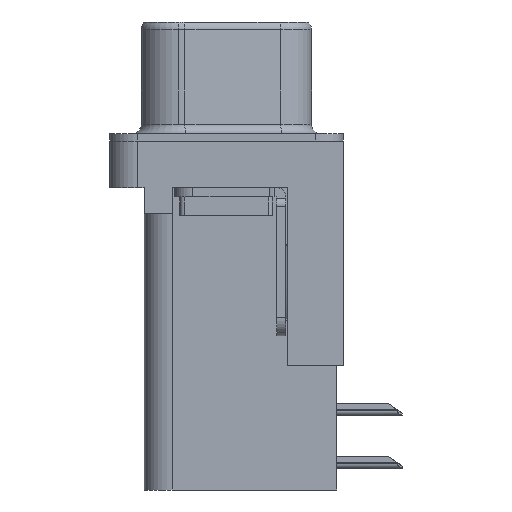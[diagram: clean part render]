
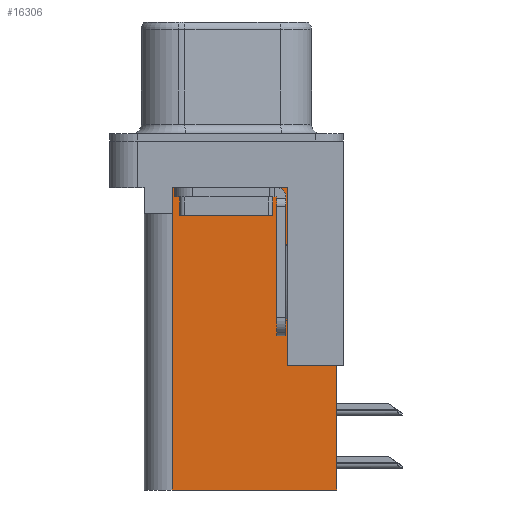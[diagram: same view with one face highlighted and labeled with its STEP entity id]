
A CAD part, left-side view. The second image highlights one B-rep face of the part: STEP entity #16306.
In plain terms, the highlighted planar face has unit normal (-1, 0, 0).
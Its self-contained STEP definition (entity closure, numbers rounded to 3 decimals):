
#5 = CARTESIAN_POINT ( 'NONE',  ( 3.7, -3.295, -18.76 ) ) ;
#32 = ORIENTED_EDGE ( 'NONE', *, *, #1229, .F. ) ;
#220 = ORIENTED_EDGE ( 'NONE', *, *, #6097, .T. ) ;
#308 = VERTEX_POINT ( 'NONE', #11061 ) ;
#889 = VERTEX_POINT ( 'NONE', #10891 ) ;
#1229 = EDGE_CURVE ( 'NONE', #1233, #20157, #14861, .T. ) ;
#1233 = VERTEX_POINT ( 'NONE', #16922 ) ;
#1778 = VERTEX_POINT ( 'NONE', #19471 ) ;
#2435 = DIRECTION ( 'NONE',  ( 0., 0., -1. ) ) ;
#2873 = DIRECTION ( 'NONE',  ( 0., 1., 0. ) ) ;
#2878 = VECTOR ( 'NONE', #2435, 1000. ) ;
#3005 = LINE ( 'NONE', #23291, #2878 ) ;
#3459 = CARTESIAN_POINT ( 'NONE',  ( 3.7, 2.925, -18.76 ) ) ;
#4246 = DIRECTION ( 'NONE',  ( 0., 1., 0. ) ) ;
#4630 = CARTESIAN_POINT ( 'NONE',  ( 3.7, -5.925, -18.76 ) ) ;
#5205 = VECTOR ( 'NONE', #12821, 1000. ) ;
#6097 = EDGE_CURVE ( 'NONE', #1233, #308, #6767, .T. ) ;
#6763 = VECTOR ( 'NONE', #7307, 1000. ) ;
#6767 = LINE ( 'NONE', #13098, #6763 ) ;
#7030 = ORIENTED_EDGE ( 'NONE', *, *, #12624, .T. ) ;
#7238 = DIRECTION ( 'NONE',  ( 0., 1., 0. ) ) ;
#7307 = DIRECTION ( 'NONE',  ( 0., 1., 0. ) ) ;
#7654 = CARTESIAN_POINT ( 'NONE',  ( 3.7, 2.925, -18.76 ) ) ;
#9260 = CARTESIAN_POINT ( 'NONE',  ( 3.7, 2.925, -3.9 ) ) ;
#9884 = ORIENTED_EDGE ( 'NONE', *, *, #19388, .T. ) ;
#10268 = VERTEX_POINT ( 'NONE', #9260 ) ;
#10859 = ORIENTED_EDGE ( 'NONE', *, *, #14201, .T. ) ;
#10891 = CARTESIAN_POINT ( 'NONE',  ( 3.7, 2.895, -2.5 ) ) ;
#11061 = CARTESIAN_POINT ( 'NONE',  ( 3.7, -3.295, -12.05 ) ) ;
#11160 = CARTESIAN_POINT ( 'NONE',  ( 3.7, -3.295, -2.5 ) ) ;
#11356 = FACE_OUTER_BOUND ( 'NONE', #13870, .T. ) ;
#11806 = DIRECTION ( 'NONE',  ( 0., 1., 0. ) ) ;
#12185 = CARTESIAN_POINT ( 'NONE',  ( 3.7, -3.295, -18.76 ) ) ;
#12386 = EDGE_CURVE ( 'NONE', #24556, #10268, #24076, .T. ) ;
#12592 = DIRECTION ( 'NONE',  ( 0., 0., 1. ) ) ;
#12624 = EDGE_CURVE ( 'NONE', #16472, #889, #23000, .T. ) ;
#12821 = DIRECTION ( 'NONE',  ( 0., 0., -1. ) ) ;
#13098 = CARTESIAN_POINT ( 'NONE',  ( 3.7, -6.295, -12.05 ) ) ;
#13870 = EDGE_LOOP ( 'NONE', ( #7030, #9884, #10859, #19218, #21485, #32, #220, #14213 ) ) ;
#14201 = EDGE_CURVE ( 'NONE', #1778, #10268, #17069, .T. ) ;
#14213 = ORIENTED_EDGE ( 'NONE', *, *, #21767, .T. ) ;
#14412 = EDGE_CURVE ( 'NONE', #20157, #24556, #16331, .T. ) ;
#14534 = DIRECTION ( 'NONE',  ( 1., 0., 0. ) ) ;
#14630 = CARTESIAN_POINT ( 'NONE',  ( 3.7, -5.925, -2. ) ) ;
#14861 = LINE ( 'NONE', #14630, #5205 ) ;
#15081 = DIRECTION ( 'NONE',  ( 0., 0., 1. ) ) ;
#15357 = AXIS2_PLACEMENT_3D ( 'NONE', #21843, #14534, #2873 ) ;
#15764 = CARTESIAN_POINT ( 'NONE',  ( 3.7, -3.295, -2.5 ) ) ;
#16281 = VECTOR ( 'NONE', #11806, 1000. ) ;
#16306 = ADVANCED_FACE ( 'NONE', ( #11356 ), #23682, .F. ) ;
#16331 = LINE ( 'NONE', #5, #16281 ) ;
#16472 = VERTEX_POINT ( 'NONE', #11160 ) ;
#16795 = CARTESIAN_POINT ( 'NONE',  ( 3.7, 0., -3.9 ) ) ;
#16922 = CARTESIAN_POINT ( 'NONE',  ( 3.7, -5.925, -12.05 ) ) ;
#17015 = VECTOR ( 'NONE', #7238, 1000. ) ;
#17069 = LINE ( 'NONE', #16795, #17015 ) ;
#19218 = ORIENTED_EDGE ( 'NONE', *, *, #12386, .F. ) ;
#19388 = EDGE_CURVE ( 'NONE', #889, #1778, #3005, .T. ) ;
#19471 = CARTESIAN_POINT ( 'NONE',  ( 3.7, 2.895, -3.9 ) ) ;
#20157 = VERTEX_POINT ( 'NONE', #4630 ) ;
#20726 = VECTOR ( 'NONE', #12592, 1000. ) ;
#20754 = LINE ( 'NONE', #12185, #20726 ) ;
#21485 = ORIENTED_EDGE ( 'NONE', *, *, #14412, .F. ) ;
#21767 = EDGE_CURVE ( 'NONE', #308, #16472, #20754, .T. ) ;
#21843 = CARTESIAN_POINT ( 'NONE',  ( 3.7, -3.295, -18.76 ) ) ;
#22951 = VECTOR ( 'NONE', #4246, 1000. ) ;
#23000 = LINE ( 'NONE', #15764, #22951 ) ;
#23291 = CARTESIAN_POINT ( 'NONE',  ( 3.7, 2.895, -3.9 ) ) ;
#23682 = PLANE ( 'NONE',  #15357 ) ;
#24034 = VECTOR ( 'NONE', #15081, 1000. ) ;
#24076 = LINE ( 'NONE', #3459, #24034 ) ;
#24556 = VERTEX_POINT ( 'NONE', #7654 ) ;
